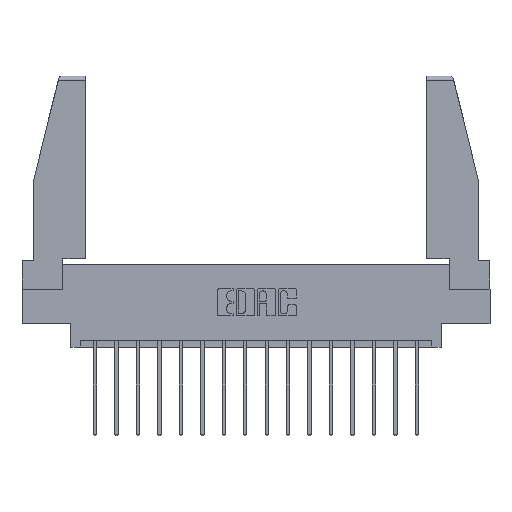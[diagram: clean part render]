
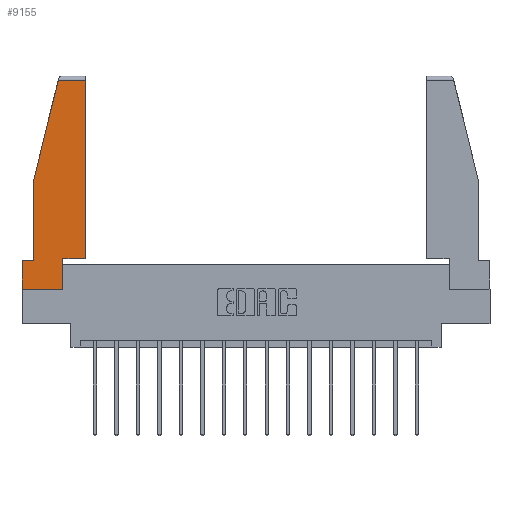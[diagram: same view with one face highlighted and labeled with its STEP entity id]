
A CAD part, top view. The second image highlights one B-rep face of the part: STEP entity #9155.
In plain terms, the highlighted planar face has unit normal (0, 0, 1).
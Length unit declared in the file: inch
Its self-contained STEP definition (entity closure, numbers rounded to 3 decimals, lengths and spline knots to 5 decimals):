
#6 = CARTESIAN_POINT ( 'NONE',  ( 0.297, 0.223, 0. ) ) ;
#261 = CARTESIAN_POINT ( 'NONE',  ( 0.297, 0.223, 0. ) ) ;
#278 = EDGE_CURVE ( 'NONE', #10890, #13833, #16972, .T. ) ;
#1336 = VECTOR ( 'NONE', #9626, 39.37008 ) ;
#1364 = CARTESIAN_POINT ( 'NONE',  ( 0.461, 1.52, 0. ) ) ;
#1382 = EDGE_CURVE ( 'NONE', #9840, #7021, #13336, .T. ) ;
#1712 = VECTOR ( 'NONE', #14874, 39.37008 ) ;
#1920 = DIRECTION ( 'NONE',  ( -1., 0., 0. ) ) ;
#2209 = FACE_OUTER_BOUND ( 'NONE', #10270, .T. ) ;
#2864 = DIRECTION ( 'NONE',  ( 1., 0., 0. ) ) ;
#3080 = VERTEX_POINT ( 'NONE', #261 ) ;
#3228 = ORIENTED_EDGE ( 'NONE', *, *, #4541, .T. ) ;
#3476 = LINE ( 'NONE', #6514, #1712 ) ;
#3710 = VECTOR ( 'NONE', #18126, 39.37008 ) ;
#3834 = CARTESIAN_POINT ( 'NONE',  ( 0.086, 0.8, 0. ) ) ;
#4035 = ORIENTED_EDGE ( 'NONE', *, *, #14554, .T. ) ;
#4322 = VERTEX_POINT ( 'NONE', #5948 ) ;
#4520 = CARTESIAN_POINT ( 'NONE',  ( 0., 0.21, 0. ) ) ;
#4541 = EDGE_CURVE ( 'NONE', #9767, #10890, #8612, .T. ) ;
#4545 = DIRECTION ( 'NONE',  ( 0., -1., 0. ) ) ;
#4663 = CARTESIAN_POINT ( 'NONE',  ( 0.086, 0.8, 0. ) ) ;
#5088 = LINE ( 'NONE', #5266, #1336 ) ;
#5183 = LINE ( 'NONE', #6, #16066 ) ;
#5266 = CARTESIAN_POINT ( 'NONE',  ( 0.461, 0.223, 0. ) ) ;
#5382 = CARTESIAN_POINT ( 'NONE',  ( 0., 0., 0. ) ) ;
#5557 = DIRECTION ( 'NONE',  ( 1., 0., 0. ) ) ;
#5696 = ORIENTED_EDGE ( 'NONE', *, *, #15705, .T. ) ;
#5771 = ORIENTED_EDGE ( 'NONE', *, *, #5874, .T. ) ;
#5874 = EDGE_CURVE ( 'NONE', #7021, #3080, #7252, .T. ) ;
#5948 = CARTESIAN_POINT ( 'NONE',  ( 0.2636, 1.52, 0. ) ) ;
#5958 = VECTOR ( 'NONE', #4545, 39.37008 ) ;
#6514 = CARTESIAN_POINT ( 'NONE',  ( 0.271, 1.55, 0. ) ) ;
#6601 = CARTESIAN_POINT ( 'NONE',  ( 0.297, 0., 0. ) ) ;
#6675 = CARTESIAN_POINT ( 'NONE',  ( 0.461, 0.223, 0. ) ) ;
#7018 = CARTESIAN_POINT ( 'NONE',  ( 0., 0.21, 0. ) ) ;
#7021 = VERTEX_POINT ( 'NONE', #9809 ) ;
#7252 = LINE ( 'NONE', #6601, #3710 ) ;
#7659 = VECTOR ( 'NONE', #1920, 39.37008 ) ;
#8255 = DIRECTION ( 'NONE',  ( 0., -1., 0. ) ) ;
#8612 = LINE ( 'NONE', #4663, #5958 ) ;
#8723 = VECTOR ( 'NONE', #8255, 39.37008 ) ;
#9053 = DIRECTION ( 'NONE',  ( 0., 0., 1. ) ) ;
#9155 = ADVANCED_FACE ( 'NONE', ( #2209 ), #17221, .T. ) ;
#9253 = ORIENTED_EDGE ( 'NONE', *, *, #278, .T. ) ;
#9339 = EDGE_CURVE ( 'NONE', #11067, #14984, #5088, .T. ) ;
#9439 = ORIENTED_EDGE ( 'NONE', *, *, #1382, .T. ) ;
#9626 = DIRECTION ( 'NONE',  ( 0., 1., 0. ) ) ;
#9767 = VERTEX_POINT ( 'NONE', #3834 ) ;
#9809 = CARTESIAN_POINT ( 'NONE',  ( 0.297, 0., 0. ) ) ;
#9840 = VERTEX_POINT ( 'NONE', #12841 ) ;
#10045 = VECTOR ( 'NONE', #16360, 39.37008 ) ;
#10270 = EDGE_LOOP ( 'NONE', ( #15679, #14901, #4035, #3228, #9253, #13957, #9439, #5771, #5696 ) ) ;
#10890 = VERTEX_POINT ( 'NONE', #16155 ) ;
#11067 = VERTEX_POINT ( 'NONE', #6675 ) ;
#11596 = EDGE_CURVE ( 'NONE', #13833, #9840, #12481, .T. ) ;
#11942 = CARTESIAN_POINT ( 'NONE',  ( 0., 1.52, 0. ) ) ;
#12481 = LINE ( 'NONE', #7018, #8723 ) ;
#12841 = CARTESIAN_POINT ( 'NONE',  ( 0., 0., 0. ) ) ;
#13336 = LINE ( 'NONE', #13903, #18017 ) ;
#13416 = AXIS2_PLACEMENT_3D ( 'NONE', #5382, #9053, #17780 ) ;
#13833 = VERTEX_POINT ( 'NONE', #17498 ) ;
#13903 = CARTESIAN_POINT ( 'NONE',  ( 0., 0., 0. ) ) ;
#13957 = ORIENTED_EDGE ( 'NONE', *, *, #11596, .T. ) ;
#14554 = EDGE_CURVE ( 'NONE', #4322, #9767, #3476, .T. ) ;
#14874 = DIRECTION ( 'NONE',  ( -0.239, -0.971, 0. ) ) ;
#14901 = ORIENTED_EDGE ( 'NONE', *, *, #16561, .T. ) ;
#14984 = VERTEX_POINT ( 'NONE', #1364 ) ;
#15157 = LINE ( 'NONE', #11942, #10045 ) ;
#15679 = ORIENTED_EDGE ( 'NONE', *, *, #9339, .T. ) ;
#15705 = EDGE_CURVE ( 'NONE', #3080, #11067, #5183, .T. ) ;
#16066 = VECTOR ( 'NONE', #2864, 39.37008 ) ;
#16155 = CARTESIAN_POINT ( 'NONE',  ( 0.086, 0.21, 0. ) ) ;
#16360 = DIRECTION ( 'NONE',  ( -1., 0., 0. ) ) ;
#16561 = EDGE_CURVE ( 'NONE', #14984, #4322, #15157, .T. ) ;
#16972 = LINE ( 'NONE', #4520, #7659 ) ;
#17221 = PLANE ( 'NONE',  #13416 ) ;
#17498 = CARTESIAN_POINT ( 'NONE',  ( 0., 0.21, 0. ) ) ;
#17780 = DIRECTION ( 'NONE',  ( 1., 0., 0. ) ) ;
#18017 = VECTOR ( 'NONE', #5557, 39.37008 ) ;
#18126 = DIRECTION ( 'NONE',  ( 0., 1., 0. ) ) ;
